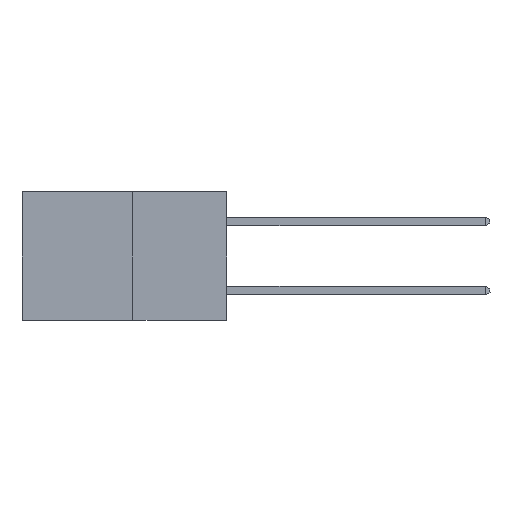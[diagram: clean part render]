
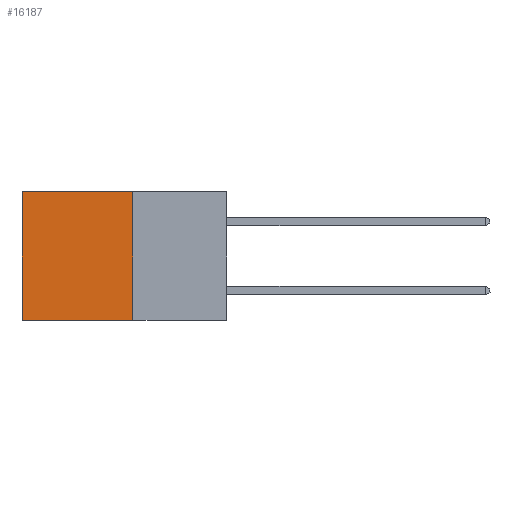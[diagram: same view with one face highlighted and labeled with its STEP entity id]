
A CAD part, left-side view. The second image highlights one B-rep face of the part: STEP entity #16187.
In plain terms, the highlighted planar face has unit normal (-1, 0, 0).
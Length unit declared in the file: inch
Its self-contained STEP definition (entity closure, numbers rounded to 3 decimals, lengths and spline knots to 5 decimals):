
#207 = EDGE_CURVE ( 'NONE', #11544, #19178, #4136, .T. ) ;
#2046 = EDGE_CURVE ( 'NONE', #11544, #19243, #15997, .T. ) ;
#2865 = CARTESIAN_POINT ( 'NONE',  ( 0.277, 0.59, 0. ) ) ;
#4059 = ORIENTED_EDGE ( 'NONE', *, *, #2046, .T. ) ;
#4136 = LINE ( 'NONE', #5527, #20952 ) ;
#4428 = DIRECTION ( 'NONE',  ( 0., 1., 0. ) ) ;
#5527 = CARTESIAN_POINT ( 'NONE',  ( 0.277, 0.27, -0.37 ) ) ;
#5787 = VECTOR ( 'NONE', #13881, 39.37008 ) ;
#6355 = ORIENTED_EDGE ( 'NONE', *, *, #18808, .T. ) ;
#6392 = DIRECTION ( 'NONE',  ( 1., 0., 0. ) ) ;
#7236 = CARTESIAN_POINT ( 'NONE',  ( 0.277, 0.27, -0.37 ) ) ;
#8547 = AXIS2_PLACEMENT_3D ( 'NONE', #12981, #6392, #17907 ) ;
#9708 = CARTESIAN_POINT ( 'NONE',  ( 0.277, 0.27, 0. ) ) ;
#10044 = ORIENTED_EDGE ( 'NONE', *, *, #14702, .F. ) ;
#10251 = LINE ( 'NONE', #7236, #5787 ) ;
#11544 = VERTEX_POINT ( 'NONE', #13728 ) ;
#11863 = CARTESIAN_POINT ( 'NONE',  ( 0.277, 0.59, -0.37 ) ) ;
#11936 = DIRECTION ( 'NONE',  ( 0., 0., -1. ) ) ;
#12981 = CARTESIAN_POINT ( 'NONE',  ( 0.277, 0.27, -0.37 ) ) ;
#13423 = ORIENTED_EDGE ( 'NONE', *, *, #207, .F. ) ;
#13728 = CARTESIAN_POINT ( 'NONE',  ( 0.277, 0.27, 0. ) ) ;
#13881 = DIRECTION ( 'NONE',  ( 0., 1., 0. ) ) ;
#13911 = CARTESIAN_POINT ( 'NONE',  ( 0.277, 0.59, -0.37 ) ) ;
#14702 = EDGE_CURVE ( 'NONE', #19178, #18497, #10251, .T. ) ;
#14950 = DIRECTION ( 'NONE',  ( 0., 0., -1. ) ) ;
#15997 = LINE ( 'NONE', #9708, #20209 ) ;
#16187 = ADVANCED_FACE ( 'NONE', ( #20681 ), #16276, .F. ) ;
#16276 = PLANE ( 'NONE',  #8547 ) ;
#16431 = EDGE_LOOP ( 'NONE', ( #6355, #10044, #13423, #4059 ) ) ;
#16920 = VECTOR ( 'NONE', #11936, 39.37008 ) ;
#17610 = CARTESIAN_POINT ( 'NONE',  ( 0.277, 0.27, -0.37 ) ) ;
#17907 = DIRECTION ( 'NONE',  ( 0., 0., -1. ) ) ;
#18497 = VERTEX_POINT ( 'NONE', #13911 ) ;
#18808 = EDGE_CURVE ( 'NONE', #19243, #18497, #20583, .T. ) ;
#19178 = VERTEX_POINT ( 'NONE', #17610 ) ;
#19243 = VERTEX_POINT ( 'NONE', #2865 ) ;
#20209 = VECTOR ( 'NONE', #4428, 39.37008 ) ;
#20583 = LINE ( 'NONE', #11863, #16920 ) ;
#20681 = FACE_OUTER_BOUND ( 'NONE', #16431, .T. ) ;
#20952 = VECTOR ( 'NONE', #14950, 39.37008 ) ;
